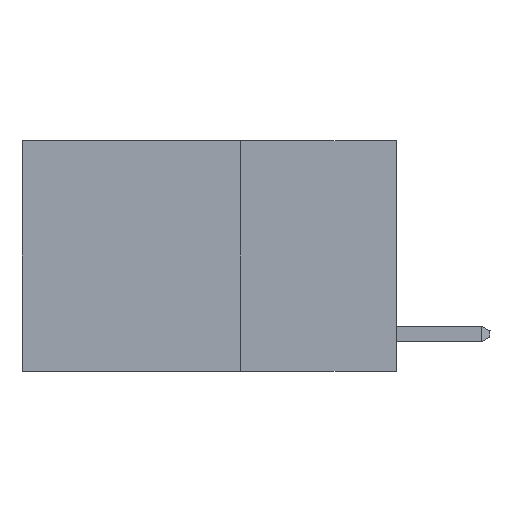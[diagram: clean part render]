
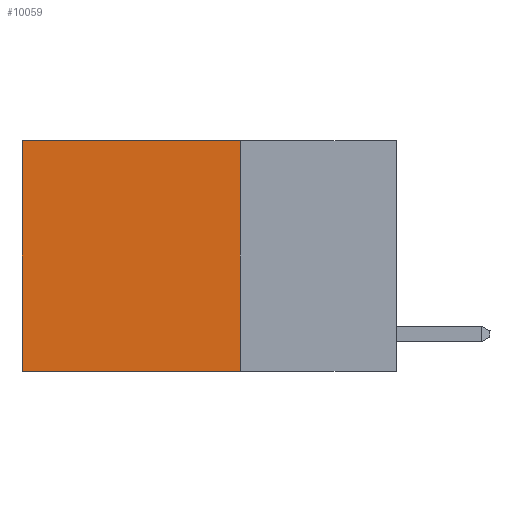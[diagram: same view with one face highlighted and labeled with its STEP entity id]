
A CAD part, left-side view. The second image highlights one B-rep face of the part: STEP entity #10059.
In plain terms, the highlighted planar face has unit normal (-1, 0, 0).
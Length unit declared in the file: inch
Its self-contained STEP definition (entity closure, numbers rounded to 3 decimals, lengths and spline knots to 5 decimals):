
#99 = DIRECTION ( 'NONE',  ( 0., 0., -1. ) ) ;
#289 = FACE_OUTER_BOUND ( 'NONE', #612, .T. ) ;
#612 = EDGE_LOOP ( 'NONE', ( #5593, #12557, #14376, #4139 ) ) ;
#978 = VECTOR ( 'NONE', #99, 39.37008 ) ;
#1118 = DIRECTION ( 'NONE',  ( 1., 0., 0. ) ) ;
#2176 = LINE ( 'NONE', #3848, #8741 ) ;
#2241 = DIRECTION ( 'NONE',  ( 0., 0., -1. ) ) ;
#2896 = AXIS2_PLACEMENT_3D ( 'NONE', #4538, #1118, #2241 ) ;
#3848 = CARTESIAN_POINT ( 'NONE',  ( 0.2625, 0.25, 0. ) ) ;
#4025 = CARTESIAN_POINT ( 'NONE',  ( 0.2625, 0.25, -0.37 ) ) ;
#4139 = ORIENTED_EDGE ( 'NONE', *, *, #4970, .T. ) ;
#4454 = CARTESIAN_POINT ( 'NONE',  ( 0.2625, 0.6, -0.37 ) ) ;
#4538 = CARTESIAN_POINT ( 'NONE',  ( 0.2625, 0.25, 0. ) ) ;
#4970 = EDGE_CURVE ( 'NONE', #11359, #13976, #2176, .T. ) ;
#5178 = LINE ( 'NONE', #11698, #6789 ) ;
#5593 = ORIENTED_EDGE ( 'NONE', *, *, #7064, .T. ) ;
#6474 = DIRECTION ( 'NONE',  ( 0., 1., 0. ) ) ;
#6789 = VECTOR ( 'NONE', #8217, 39.37008 ) ;
#6858 = CARTESIAN_POINT ( 'NONE',  ( 0.2625, 0.25, 0. ) ) ;
#7064 = EDGE_CURVE ( 'NONE', #13976, #12110, #11485, .T. ) ;
#8217 = DIRECTION ( 'NONE',  ( 0., 1., 0. ) ) ;
#8499 = CARTESIAN_POINT ( 'NONE',  ( 0.2625, 0.6, 0. ) ) ;
#8741 = VECTOR ( 'NONE', #6474, 39.37008 ) ;
#9817 = LINE ( 'NONE', #6858, #978 ) ;
#9866 = VERTEX_POINT ( 'NONE', #4025 ) ;
#10059 = ADVANCED_FACE ( 'NONE', ( #289 ), #13601, .F. ) ;
#10181 = DIRECTION ( 'NONE',  ( 0., 0., -1. ) ) ;
#10316 = EDGE_CURVE ( 'NONE', #11359, #9866, #9817, .T. ) ;
#11359 = VERTEX_POINT ( 'NONE', #11684 ) ;
#11485 = LINE ( 'NONE', #12407, #12214 ) ;
#11684 = CARTESIAN_POINT ( 'NONE',  ( 0.2625, 0.25, 0. ) ) ;
#11698 = CARTESIAN_POINT ( 'NONE',  ( 0.2625, 0.25, -0.37 ) ) ;
#12110 = VERTEX_POINT ( 'NONE', #4454 ) ;
#12214 = VECTOR ( 'NONE', #10181, 39.37008 ) ;
#12407 = CARTESIAN_POINT ( 'NONE',  ( 0.2625, 0.6, 0. ) ) ;
#12557 = ORIENTED_EDGE ( 'NONE', *, *, #14462, .F. ) ;
#13601 = PLANE ( 'NONE',  #2896 ) ;
#13976 = VERTEX_POINT ( 'NONE', #8499 ) ;
#14376 = ORIENTED_EDGE ( 'NONE', *, *, #10316, .F. ) ;
#14462 = EDGE_CURVE ( 'NONE', #9866, #12110, #5178, .T. ) ;
